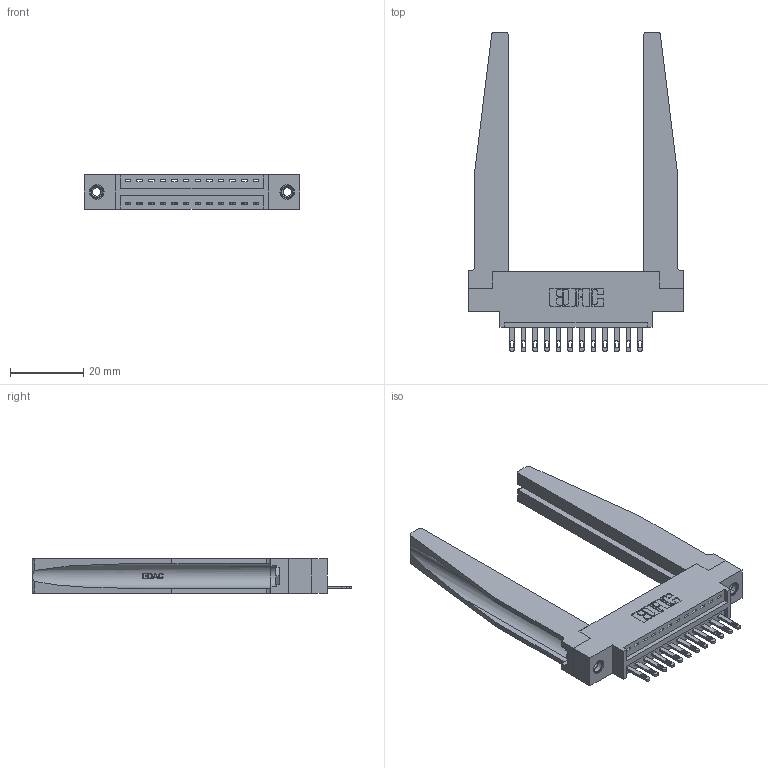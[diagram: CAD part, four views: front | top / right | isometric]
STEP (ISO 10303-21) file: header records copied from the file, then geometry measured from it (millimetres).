
FILE_DESCRIPTION (( 'STEP AP203' ), '1' );
FILE_NAME ('346-012-500-678.STEP', '2022-05-05T02:14:47', ( '' ), ( '' ), 'SwSTEP 2.0', 'SolidWorks 2020', '' );
FILE_SCHEMA (( 'CONFIG_CONTROL_DESIGN' ));
Length unit declared in the file: inch
Products named in the file (5): 346 Part_0.170 Offset - 0.156 Dia-TH; 346-012-500-678; 345-250-001_345-250-001-102; 345-292-001_345-293-100; 346-220-078_345-220-078
Assembly tree (17 placements, depth 2):
  346-012-500-678
    346 Part_0.170 Offset - 0.156 Dia-TH
    345-292-001_345-293-100  x12
    346-220-078_345-220-078  x2
    345-250-001_345-250-001-102  x2
Bounding box: 58.67 x 87.12 x 9.4 mm (x, y, z)
Volume: 12153.3 mm3; surface area: 12991.8 mm2
Topology: 17 solids, 17 shells, 1022 faces, 3001 edges, 1990 vertices
Faces by surface type: plane 644, cylinder 326, bspline 36, cone 12, torus 4
Entity records: 16712 total; most frequent: CARTESIAN_POINT 3789, ORIENTED_EDGE 2622, DIRECTION 2365, EDGE_CURVE 1311, VECTOR 1033, LINE 1033, VERTEX_POINT 868, AXIS2_PLACEMENT_3D 666
